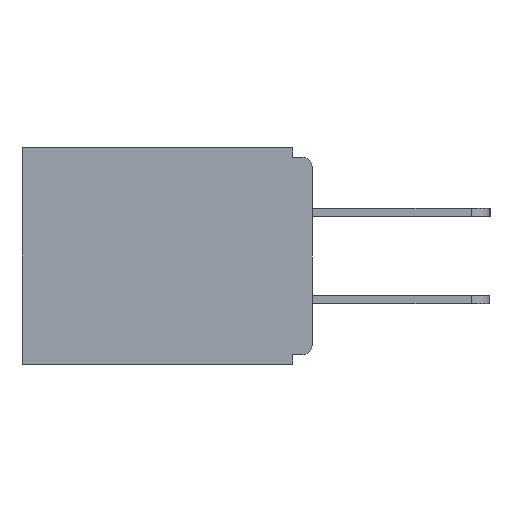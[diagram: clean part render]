
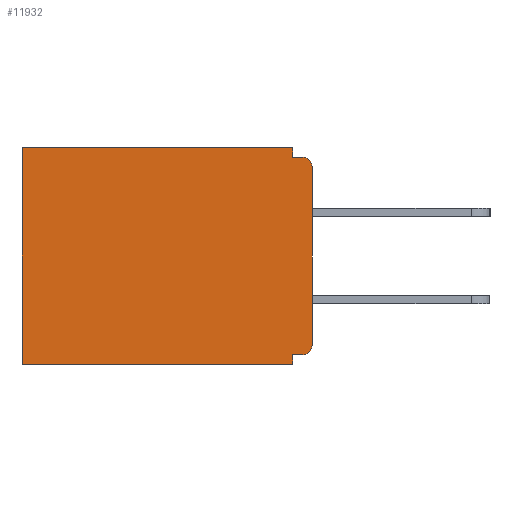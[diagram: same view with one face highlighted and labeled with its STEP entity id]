
A CAD part, left-side view. The second image highlights one B-rep face of the part: STEP entity #11932.
In plain terms, the highlighted planar face has unit normal (-1, 0, 0).
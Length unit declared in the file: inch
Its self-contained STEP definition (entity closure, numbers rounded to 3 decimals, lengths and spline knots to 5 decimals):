
#687 = EDGE_CURVE ( 'NONE', #15904, #20327, #21018, .T. ) ;
#691 = VECTOR ( 'NONE', #21969, 39.37008 ) ;
#706 = AXIS2_PLACEMENT_3D ( 'NONE', #9698, #21619, #17935 ) ;
#1085 = CARTESIAN_POINT ( 'NONE',  ( 0.298, 0., -0.343 ) ) ;
#1146 = VERTEX_POINT ( 'NONE', #4120 ) ;
#1207 = VERTEX_POINT ( 'NONE', #19676 ) ;
#1234 = DIRECTION ( 'NONE',  ( 0., 0., -1. ) ) ;
#1239 = CARTESIAN_POINT ( 'NONE',  ( 0.298, 0., 0. ) ) ;
#1259 = AXIS2_PLACEMENT_3D ( 'NONE', #19704, #5946, #7719 ) ;
#1608 = DIRECTION ( 'NONE',  ( -1., 0., 0. ) ) ;
#2123 = AXIS2_PLACEMENT_3D ( 'NONE', #3254, #1608, #16817 ) ;
#2366 = EDGE_CURVE ( 'NONE', #1146, #18424, #18479, .T. ) ;
#2393 = EDGE_CURVE ( 'NONE', #9465, #4076, #20679, .T. ) ;
#2829 = CARTESIAN_POINT ( 'NONE',  ( 0.298, 0.031, -0.015 ) ) ;
#2843 = VECTOR ( 'NONE', #16592, 39.37008 ) ;
#3041 = EDGE_CURVE ( 'NONE', #15904, #4076, #9958, .T. ) ;
#3254 = CARTESIAN_POINT ( 'NONE',  ( 0.298, 0.015, -0.03 ) ) ;
#4076 = VERTEX_POINT ( 'NONE', #10995 ) ;
#4120 = CARTESIAN_POINT ( 'NONE',  ( 0.298, 0.46, 0. ) ) ;
#4385 = VECTOR ( 'NONE', #21015, 39.37008 ) ;
#4443 = PLANE ( 'NONE',  #1259 ) ;
#4681 = DIRECTION ( 'NONE',  ( 0., 0., -1. ) ) ;
#5324 = EDGE_CURVE ( 'NONE', #17591, #9748, #16386, .T. ) ;
#5677 = ORIENTED_EDGE ( 'NONE', *, *, #8876, .F. ) ;
#5946 = DIRECTION ( 'NONE',  ( 1., 0., 0. ) ) ;
#7222 = LINE ( 'NONE', #7752, #15513 ) ;
#7330 = EDGE_CURVE ( 'NONE', #9465, #8507, #7222, .T. ) ;
#7430 = ORIENTED_EDGE ( 'NONE', *, *, #7330, .F. ) ;
#7458 = LINE ( 'NONE', #1085, #2843 ) ;
#7719 = DIRECTION ( 'NONE',  ( 0., 0., -1. ) ) ;
#7752 = CARTESIAN_POINT ( 'NONE',  ( 0.298, 0., -0.328 ) ) ;
#8507 = VERTEX_POINT ( 'NONE', #13317 ) ;
#8876 = EDGE_CURVE ( 'NONE', #1207, #18424, #7458, .T. ) ;
#9465 = VERTEX_POINT ( 'NONE', #16788 ) ;
#9625 = DIRECTION ( 'NONE',  ( 0., 0., -1. ) ) ;
#9698 = CARTESIAN_POINT ( 'NONE',  ( 0.298, 0.015, -0.313 ) ) ;
#9748 = VERTEX_POINT ( 'NONE', #2829 ) ;
#9958 = LINE ( 'NONE', #1239, #14457 ) ;
#10401 = CARTESIAN_POINT ( 'NONE',  ( 0.298, 0.46, -0.343 ) ) ;
#10995 = CARTESIAN_POINT ( 'NONE',  ( 0.298, 0., -0.313 ) ) ;
#11315 = EDGE_CURVE ( 'NONE', #9748, #20327, #16577, .T. ) ;
#11316 = VECTOR ( 'NONE', #9625, 39.37008 ) ;
#11932 = ADVANCED_FACE ( 'NONE', ( #20573 ), #4443, .F. ) ;
#12044 = VECTOR ( 'NONE', #19974, 39.37008 ) ;
#12659 = EDGE_CURVE ( 'NONE', #17591, #1146, #19167, .T. ) ;
#12959 = CARTESIAN_POINT ( 'NONE',  ( 0.298, 0.46, 0. ) ) ;
#12971 = LINE ( 'NONE', #14124, #4385 ) ;
#13317 = CARTESIAN_POINT ( 'NONE',  ( 0.298, 0.031, -0.328 ) ) ;
#14124 = CARTESIAN_POINT ( 'NONE',  ( 0.298, 0.031, -0.343 ) ) ;
#14457 = VECTOR ( 'NONE', #4681, 39.37008 ) ;
#14654 = EDGE_CURVE ( 'NONE', #8507, #1207, #12971, .T. ) ;
#14894 = ORIENTED_EDGE ( 'NONE', *, *, #11315, .F. ) ;
#15513 = VECTOR ( 'NONE', #19661, 39.37008 ) ;
#15904 = VERTEX_POINT ( 'NONE', #21617 ) ;
#16386 = LINE ( 'NONE', #20100, #18485 ) ;
#16546 = CARTESIAN_POINT ( 'NONE',  ( 0.298, 0., -0.015 ) ) ;
#16577 = LINE ( 'NONE', #16546, #12044 ) ;
#16592 = DIRECTION ( 'NONE',  ( 0., 1., 0. ) ) ;
#16682 = ORIENTED_EDGE ( 'NONE', *, *, #687, .T. ) ;
#16788 = CARTESIAN_POINT ( 'NONE',  ( 0.298, 0.015, -0.328 ) ) ;
#16817 = DIRECTION ( 'NONE',  ( 0., 0., -1. ) ) ;
#16822 = CARTESIAN_POINT ( 'NONE',  ( 0.298, 0., 0. ) ) ;
#17282 = ORIENTED_EDGE ( 'NONE', *, *, #2366, .T. ) ;
#17385 = ORIENTED_EDGE ( 'NONE', *, *, #3041, .F. ) ;
#17568 = ORIENTED_EDGE ( 'NONE', *, *, #14654, .F. ) ;
#17591 = VERTEX_POINT ( 'NONE', #19018 ) ;
#17935 = DIRECTION ( 'NONE',  ( 0., 0., -1. ) ) ;
#18195 = ORIENTED_EDGE ( 'NONE', *, *, #5324, .F. ) ;
#18424 = VERTEX_POINT ( 'NONE', #10401 ) ;
#18479 = LINE ( 'NONE', #12959, #11316 ) ;
#18485 = VECTOR ( 'NONE', #1234, 39.37008 ) ;
#18613 = EDGE_LOOP ( 'NONE', ( #16682, #14894, #18195, #19977, #17282, #5677, #17568, #7430, #20200, #17385 ) ) ;
#19018 = CARTESIAN_POINT ( 'NONE',  ( 0.298, 0.031, 0. ) ) ;
#19083 = CARTESIAN_POINT ( 'NONE',  ( 0.298, 0.015, -0.015 ) ) ;
#19167 = LINE ( 'NONE', #16822, #691 ) ;
#19661 = DIRECTION ( 'NONE',  ( 0., 1., 0. ) ) ;
#19676 = CARTESIAN_POINT ( 'NONE',  ( 0.298, 0.031, -0.343 ) ) ;
#19704 = CARTESIAN_POINT ( 'NONE',  ( 0.298, 0., 0. ) ) ;
#19974 = DIRECTION ( 'NONE',  ( 0., -1., 0. ) ) ;
#19977 = ORIENTED_EDGE ( 'NONE', *, *, #12659, .T. ) ;
#20100 = CARTESIAN_POINT ( 'NONE',  ( 0.298, 0.031, -0.343 ) ) ;
#20200 = ORIENTED_EDGE ( 'NONE', *, *, #2393, .T. ) ;
#20327 = VERTEX_POINT ( 'NONE', #19083 ) ;
#20573 = FACE_OUTER_BOUND ( 'NONE', #18613, .T. ) ;
#20679 = CIRCLE ( 'NONE', #706, 0.015 ) ;
#21015 = DIRECTION ( 'NONE',  ( 0., 0., -1. ) ) ;
#21018 = CIRCLE ( 'NONE', #2123, 0.015 ) ;
#21617 = CARTESIAN_POINT ( 'NONE',  ( 0.298, 0., -0.03 ) ) ;
#21619 = DIRECTION ( 'NONE',  ( -1., 0., 0. ) ) ;
#21969 = DIRECTION ( 'NONE',  ( 0., 1., 0. ) ) ;
